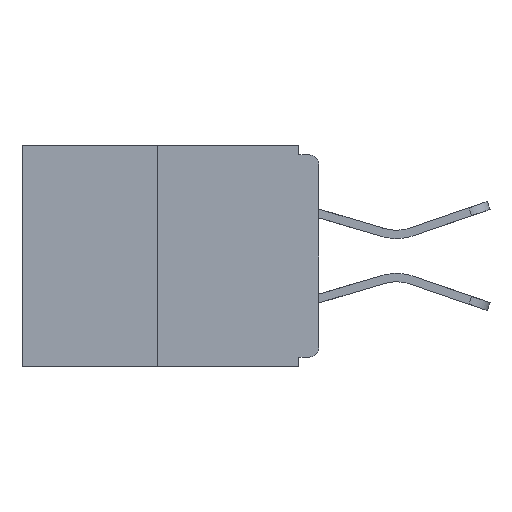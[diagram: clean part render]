
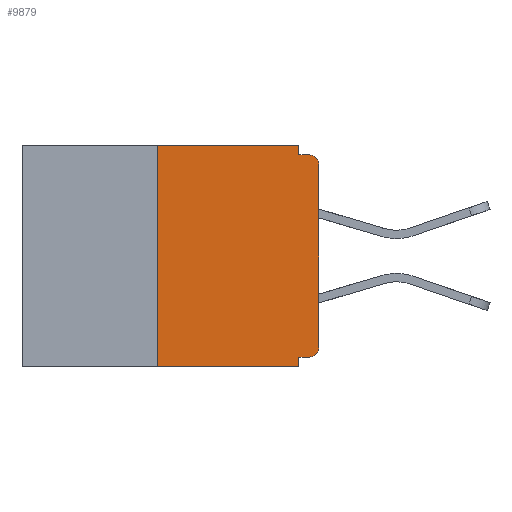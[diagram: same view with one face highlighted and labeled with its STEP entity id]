
A CAD part, left-side view. The second image highlights one B-rep face of the part: STEP entity #9879.
In plain terms, the highlighted planar face has unit normal (-1, 0, 0).
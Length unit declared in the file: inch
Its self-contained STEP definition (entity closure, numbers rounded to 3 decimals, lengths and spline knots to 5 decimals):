
#44 = CARTESIAN_POINT ( 'NONE',  ( 0., 0.46, 0. ) ) ;
#78 = CIRCLE ( 'NONE', #5689, 0.015 ) ;
#99 = ORIENTED_EDGE ( 'NONE', *, *, #12213, .F. ) ;
#140 = FACE_OUTER_BOUND ( 'NONE', #12490, .T. ) ;
#380 = VECTOR ( 'NONE', #8290, 39.37008 ) ;
#423 = LINE ( 'NONE', #1439, #4398 ) ;
#545 = CARTESIAN_POINT ( 'NONE',  ( 0., 0., 0. ) ) ;
#933 = ORIENTED_EDGE ( 'NONE', *, *, #3489, .F. ) ;
#1174 = VERTEX_POINT ( 'NONE', #6244 ) ;
#1439 = CARTESIAN_POINT ( 'NONE',  ( 0., 0.25, 0. ) ) ;
#1520 = EDGE_CURVE ( 'NONE', #4478, #2460, #4646, .T. ) ;
#1522 = DIRECTION ( 'NONE',  ( 0., 0., 1. ) ) ;
#1666 = LINE ( 'NONE', #545, #3963 ) ;
#2460 = VERTEX_POINT ( 'NONE', #2972 ) ;
#2533 = EDGE_CURVE ( 'NONE', #9653, #2460, #7226, .T. ) ;
#2719 = CARTESIAN_POINT ( 'NONE',  ( 0., 0., -0.313 ) ) ;
#2963 = LINE ( 'NONE', #4432, #380 ) ;
#2972 = CARTESIAN_POINT ( 'NONE',  ( 0., 0.031, -0.343 ) ) ;
#3236 = LINE ( 'NONE', #44, #4160 ) ;
#3365 = ORIENTED_EDGE ( 'NONE', *, *, #10310, .F. ) ;
#3380 = AXIS2_PLACEMENT_3D ( 'NONE', #7786, #3695, #6717 ) ;
#3489 = EDGE_CURVE ( 'NONE', #6236, #7485, #3236, .T. ) ;
#3695 = DIRECTION ( 'NONE',  ( 1., 0., 0. ) ) ;
#3742 = ORIENTED_EDGE ( 'NONE', *, *, #1520, .F. ) ;
#3793 = DIRECTION ( 'NONE',  ( -1., 0., 0. ) ) ;
#3963 = VECTOR ( 'NONE', #10151, 39.37008 ) ;
#4055 = DIRECTION ( 'NONE',  ( 0., -1., 0. ) ) ;
#4160 = VECTOR ( 'NONE', #7704, 39.37008 ) ;
#4227 = VERTEX_POINT ( 'NONE', #4848 ) ;
#4306 = CARTESIAN_POINT ( 'NONE',  ( 0., 0.25, -0.343 ) ) ;
#4398 = VECTOR ( 'NONE', #1522, 39.37008 ) ;
#4432 = CARTESIAN_POINT ( 'NONE',  ( 0., 0.031, 0. ) ) ;
#4478 = VERTEX_POINT ( 'NONE', #6321 ) ;
#4501 = VECTOR ( 'NONE', #8761, 39.37008 ) ;
#4507 = EDGE_CURVE ( 'NONE', #11347, #12126, #1666, .T. ) ;
#4646 = LINE ( 'NONE', #4775, #4501 ) ;
#4753 = ORIENTED_EDGE ( 'NONE', *, *, #12510, .T. ) ;
#4775 = CARTESIAN_POINT ( 'NONE',  ( 0., 0.031, -0.343 ) ) ;
#4848 = CARTESIAN_POINT ( 'NONE',  ( 0., 0.031, -0.015 ) ) ;
#4927 = AXIS2_PLACEMENT_3D ( 'NONE', #9664, #3793, #10679 ) ;
#4994 = ORIENTED_EDGE ( 'NONE', *, *, #11349, .T. ) ;
#5084 = DIRECTION ( 'NONE',  ( -1., 0., 0. ) ) ;
#5689 = AXIS2_PLACEMENT_3D ( 'NONE', #9026, #5084, #11117 ) ;
#5750 = DIRECTION ( 'NONE',  ( 0., 1., 0. ) ) ;
#6236 = VERTEX_POINT ( 'NONE', #7634 ) ;
#6244 = CARTESIAN_POINT ( 'NONE',  ( 0., 0.015, -0.328 ) ) ;
#6321 = CARTESIAN_POINT ( 'NONE',  ( 0., 0.031, -0.328 ) ) ;
#6326 = ORIENTED_EDGE ( 'NONE', *, *, #11390, .F. ) ;
#6717 = DIRECTION ( 'NONE',  ( 0., 0., -1. ) ) ;
#6781 = CARTESIAN_POINT ( 'NONE',  ( 0., 0., -0.328 ) ) ;
#6917 = ORIENTED_EDGE ( 'NONE', *, *, #4507, .T. ) ;
#7057 = VECTOR ( 'NONE', #4055, 39.37008 ) ;
#7226 = LINE ( 'NONE', #8116, #7057 ) ;
#7347 = ORIENTED_EDGE ( 'NONE', *, *, #2533, .T. ) ;
#7485 = VERTEX_POINT ( 'NONE', #11621 ) ;
#7511 = ORIENTED_EDGE ( 'NONE', *, *, #10384, .F. ) ;
#7634 = CARTESIAN_POINT ( 'NONE',  ( 0., 0.25, 0. ) ) ;
#7695 = CARTESIAN_POINT ( 'NONE',  ( 0., 0.015, -0.015 ) ) ;
#7704 = DIRECTION ( 'NONE',  ( 0., -1., 0. ) ) ;
#7786 = CARTESIAN_POINT ( 'NONE',  ( 0., 0.46, 0. ) ) ;
#7929 = VECTOR ( 'NONE', #8635, 39.37008 ) ;
#8116 = CARTESIAN_POINT ( 'NONE',  ( 0., 0.46, -0.343 ) ) ;
#8290 = DIRECTION ( 'NONE',  ( 0., 0., -1. ) ) ;
#8340 = CARTESIAN_POINT ( 'NONE',  ( 0., 0., -0.03 ) ) ;
#8380 = CIRCLE ( 'NONE', #4927, 0.015 ) ;
#8635 = DIRECTION ( 'NONE',  ( 0., -1., 0. ) ) ;
#8761 = DIRECTION ( 'NONE',  ( 0., 0., -1. ) ) ;
#9026 = CARTESIAN_POINT ( 'NONE',  ( 0., 0.015, -0.03 ) ) ;
#9321 = LINE ( 'NONE', #6781, #11484 ) ;
#9653 = VERTEX_POINT ( 'NONE', #4306 ) ;
#9664 = CARTESIAN_POINT ( 'NONE',  ( 0., 0.015, -0.313 ) ) ;
#9706 = CARTESIAN_POINT ( 'NONE',  ( 0., 0., -0.015 ) ) ;
#9879 = ADVANCED_FACE ( 'NONE', ( #140 ), #11573, .F. ) ;
#10151 = DIRECTION ( 'NONE',  ( 0., 0., 1. ) ) ;
#10310 = EDGE_CURVE ( 'NONE', #1174, #4478, #9321, .T. ) ;
#10384 = EDGE_CURVE ( 'NONE', #4227, #10862, #10581, .T. ) ;
#10581 = LINE ( 'NONE', #9706, #7929 ) ;
#10679 = DIRECTION ( 'NONE',  ( 0., 0., -1. ) ) ;
#10862 = VERTEX_POINT ( 'NONE', #7695 ) ;
#11117 = DIRECTION ( 'NONE',  ( 0., 0., -1. ) ) ;
#11347 = VERTEX_POINT ( 'NONE', #2719 ) ;
#11349 = EDGE_CURVE ( 'NONE', #1174, #11347, #8380, .T. ) ;
#11390 = EDGE_CURVE ( 'NONE', #9653, #6236, #423, .T. ) ;
#11484 = VECTOR ( 'NONE', #5750, 39.37008 ) ;
#11573 = PLANE ( 'NONE',  #3380 ) ;
#11621 = CARTESIAN_POINT ( 'NONE',  ( 0., 0.031, 0. ) ) ;
#12126 = VERTEX_POINT ( 'NONE', #8340 ) ;
#12213 = EDGE_CURVE ( 'NONE', #7485, #4227, #2963, .T. ) ;
#12490 = EDGE_LOOP ( 'NONE', ( #933, #6326, #7347, #3742, #3365, #4994, #6917, #4753, #7511, #99 ) ) ;
#12510 = EDGE_CURVE ( 'NONE', #12126, #10862, #78, .T. ) ;
